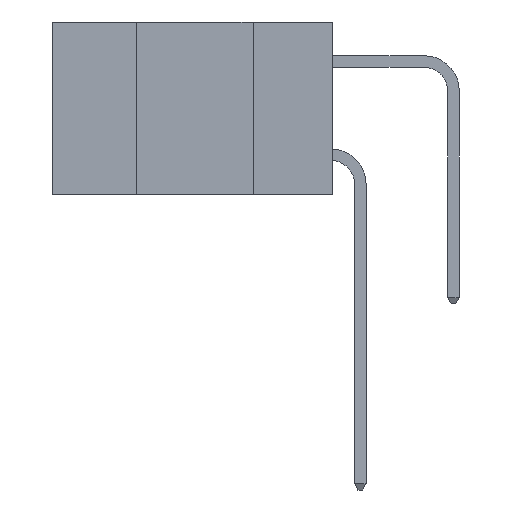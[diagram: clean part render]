
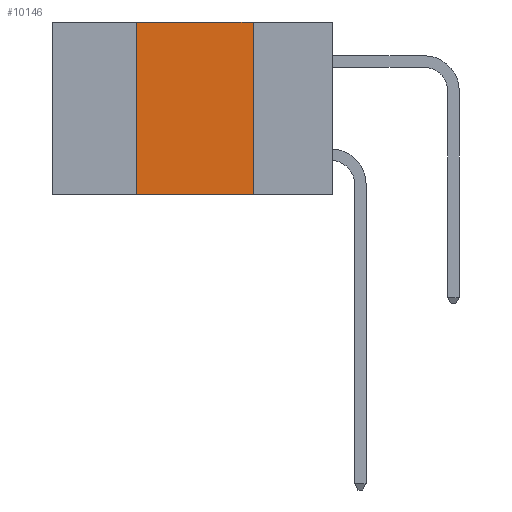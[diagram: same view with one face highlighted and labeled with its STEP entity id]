
A CAD part, left-side view. The second image highlights one B-rep face of the part: STEP entity #10146.
In plain terms, the highlighted planar face has unit normal (-1, 0, 0).
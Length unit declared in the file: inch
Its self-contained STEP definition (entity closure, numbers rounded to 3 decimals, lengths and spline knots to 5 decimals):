
#1440 = VECTOR ( 'NONE', #5828, 39.37008 ) ;
#1907 = CARTESIAN_POINT ( 'NONE',  ( 0., 0.6, 0. ) ) ;
#1949 = VERTEX_POINT ( 'NONE', #10495 ) ;
#2176 = VERTEX_POINT ( 'NONE', #12985 ) ;
#2221 = VERTEX_POINT ( 'NONE', #20637 ) ;
#3751 = DIRECTION ( 'NONE',  ( 1., 0., 0. ) ) ;
#4406 = CARTESIAN_POINT ( 'NONE',  ( 0., 0.42, 0. ) ) ;
#4751 = VERTEX_POINT ( 'NONE', #4406 ) ;
#4799 = LINE ( 'NONE', #7048, #18535 ) ;
#4906 = ORIENTED_EDGE ( 'NONE', *, *, #12400, .T. ) ;
#5828 = DIRECTION ( 'NONE',  ( 0., 0., -1. ) ) ;
#6221 = FACE_OUTER_BOUND ( 'NONE', #17350, .T. ) ;
#6338 = LINE ( 'NONE', #16461, #1440 ) ;
#6756 = CARTESIAN_POINT ( 'NONE',  ( 0., 0.42, -0.37 ) ) ;
#7048 = CARTESIAN_POINT ( 'NONE',  ( 0., 0.6, 0. ) ) ;
#7266 = LINE ( 'NONE', #22845, #16193 ) ;
#8025 = ORIENTED_EDGE ( 'NONE', *, *, #10010, .F. ) ;
#8323 = ORIENTED_EDGE ( 'NONE', *, *, #8820, .F. ) ;
#8820 = EDGE_CURVE ( 'NONE', #2221, #2176, #6338, .T. ) ;
#8856 = DIRECTION ( 'NONE',  ( 0., -1., 0. ) ) ;
#10010 = EDGE_CURVE ( 'NONE', #4751, #2221, #4799, .T. ) ;
#10146 = ADVANCED_FACE ( 'NONE', ( #6221 ), #14541, .F. ) ;
#10495 = CARTESIAN_POINT ( 'NONE',  ( 0., 0.42, -0.37 ) ) ;
#11205 = EDGE_CURVE ( 'NONE', #1949, #4751, #17653, .T. ) ;
#12400 = EDGE_CURVE ( 'NONE', #1949, #2176, #7266, .T. ) ;
#12985 = CARTESIAN_POINT ( 'NONE',  ( 0., 0.17, -0.37 ) ) ;
#13032 = AXIS2_PLACEMENT_3D ( 'NONE', #1907, #3751, #16334 ) ;
#13474 = VECTOR ( 'NONE', #21059, 39.37008 ) ;
#13902 = ORIENTED_EDGE ( 'NONE', *, *, #11205, .F. ) ;
#14541 = PLANE ( 'NONE',  #13032 ) ;
#16193 = VECTOR ( 'NONE', #19330, 39.37008 ) ;
#16334 = DIRECTION ( 'NONE',  ( 0., 0., -1. ) ) ;
#16461 = CARTESIAN_POINT ( 'NONE',  ( 0., 0.17, -0.37 ) ) ;
#17350 = EDGE_LOOP ( 'NONE', ( #8323, #8025, #13902, #4906 ) ) ;
#17653 = LINE ( 'NONE', #6756, #13474 ) ;
#18535 = VECTOR ( 'NONE', #8856, 39.37008 ) ;
#19330 = DIRECTION ( 'NONE',  ( 0., -1., 0. ) ) ;
#20637 = CARTESIAN_POINT ( 'NONE',  ( 0., 0.17, 0. ) ) ;
#21059 = DIRECTION ( 'NONE',  ( 0., 0., 1. ) ) ;
#22845 = CARTESIAN_POINT ( 'NONE',  ( 0., 0.6, -0.37 ) ) ;
